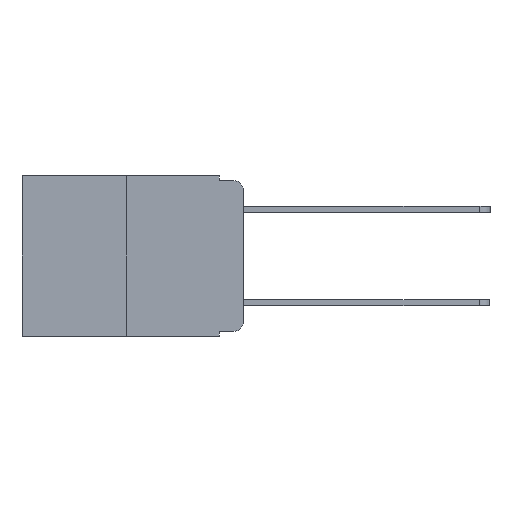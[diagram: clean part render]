
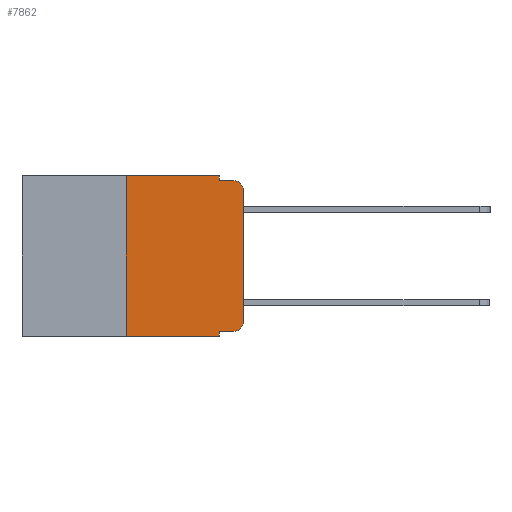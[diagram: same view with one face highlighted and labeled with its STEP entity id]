
A CAD part, left-side view. The second image highlights one B-rep face of the part: STEP entity #7862.
In plain terms, the highlighted planar face has unit normal (-1, 0, 0).
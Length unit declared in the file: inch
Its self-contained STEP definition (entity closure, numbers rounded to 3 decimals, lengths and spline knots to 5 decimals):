
#88 = ORIENTED_EDGE ( 'NONE', *, *, #5108, .T. ) ;
#132 = CARTESIAN_POINT ( 'NONE',  ( 0., 0.02, -0.01 ) ) ;
#271 = VERTEX_POINT ( 'NONE', #17676 ) ;
#285 = LINE ( 'NONE', #19377, #10182 ) ;
#403 = CARTESIAN_POINT ( 'NONE',  ( 0., 0.25, 0. ) ) ;
#944 = VECTOR ( 'NONE', #24253, 39.37008 ) ;
#967 = LINE ( 'NONE', #19892, #7755 ) ;
#1356 = CARTESIAN_POINT ( 'NONE',  ( 0., 0.051, 0. ) ) ;
#1416 = CIRCLE ( 'NONE', #23635, 0.02 ) ;
#1637 = CARTESIAN_POINT ( 'NONE',  ( 0., 0.02, -0.03 ) ) ;
#1707 = DIRECTION ( 'NONE',  ( 0., -1., 0. ) ) ;
#1805 = VERTEX_POINT ( 'NONE', #12002 ) ;
#2057 = CARTESIAN_POINT ( 'NONE',  ( 0., 0.25, -0.343 ) ) ;
#2351 = DIRECTION ( 'NONE',  ( 0., -1., 0. ) ) ;
#2490 = VERTEX_POINT ( 'NONE', #21714 ) ;
#2583 = CARTESIAN_POINT ( 'NONE',  ( 0., 0.473, 0. ) ) ;
#2915 = VERTEX_POINT ( 'NONE', #132 ) ;
#2989 = EDGE_CURVE ( 'NONE', #1805, #16256, #3990, .T. ) ;
#3214 = VERTEX_POINT ( 'NONE', #21107 ) ;
#3270 = ORIENTED_EDGE ( 'NONE', *, *, #4165, .F. ) ;
#3385 = VECTOR ( 'NONE', #1707, 39.37008 ) ;
#3662 = DIRECTION ( 'NONE',  ( 0., 0., -1. ) ) ;
#3990 = LINE ( 'NONE', #11478, #3385 ) ;
#4165 = EDGE_CURVE ( 'NONE', #3214, #9119, #20747, .T. ) ;
#4185 = AXIS2_PLACEMENT_3D ( 'NONE', #1637, #15218, #3662 ) ;
#4324 = EDGE_CURVE ( 'NONE', #1805, #4409, #967, .T. ) ;
#4409 = VERTEX_POINT ( 'NONE', #9359 ) ;
#5108 = EDGE_CURVE ( 'NONE', #10859, #2490, #285, .T. ) ;
#6042 = EDGE_LOOP ( 'NONE', ( #88, #7217, #12386, #22793, #3270, #14163, #10894, #15927, #12108, #21958 ) ) ;
#6493 = FACE_OUTER_BOUND ( 'NONE', #6042, .T. ) ;
#6657 = VECTOR ( 'NONE', #21418, 39.37008 ) ;
#6809 = DIRECTION ( 'NONE',  ( 0., 0., 1. ) ) ;
#6820 = VECTOR ( 'NONE', #2351, 39.37008 ) ;
#7139 = DIRECTION ( 'NONE',  ( 0., 0., -1. ) ) ;
#7217 = ORIENTED_EDGE ( 'NONE', *, *, #22081, .T. ) ;
#7258 = CARTESIAN_POINT ( 'NONE',  ( 0., 0.02, -0.313 ) ) ;
#7755 = VECTOR ( 'NONE', #22128, 39.37008 ) ;
#7862 = ADVANCED_FACE ( 'NONE', ( #6493 ), #19528, .F. ) ;
#9119 = VERTEX_POINT ( 'NONE', #1356 ) ;
#9254 = DIRECTION ( 'NONE',  ( 0., 0., -1. ) ) ;
#9325 = VERTEX_POINT ( 'NONE', #2057 ) ;
#9359 = CARTESIAN_POINT ( 'NONE',  ( 0., 0.051, -0.343 ) ) ;
#9386 = CARTESIAN_POINT ( 'NONE',  ( 0., 0.051, -0.01 ) ) ;
#10182 = VECTOR ( 'NONE', #6809, 39.37008 ) ;
#10185 = DIRECTION ( 'NONE',  ( 1., 0., 0. ) ) ;
#10850 = EDGE_CURVE ( 'NONE', #9325, #3214, #11871, .T. ) ;
#10859 = VERTEX_POINT ( 'NONE', #21501 ) ;
#10894 = ORIENTED_EDGE ( 'NONE', *, *, #22531, .T. ) ;
#10960 = CARTESIAN_POINT ( 'NONE',  ( 0., 0.473, -0.343 ) ) ;
#11478 = CARTESIAN_POINT ( 'NONE',  ( 0., 0.051, -0.333 ) ) ;
#11871 = LINE ( 'NONE', #403, #6657 ) ;
#12002 = CARTESIAN_POINT ( 'NONE',  ( 0., 0.051, -0.333 ) ) ;
#12108 = ORIENTED_EDGE ( 'NONE', *, *, #2989, .T. ) ;
#12386 = ORIENTED_EDGE ( 'NONE', *, *, #19630, .F. ) ;
#12399 = VECTOR ( 'NONE', #7139, 39.37008 ) ;
#14163 = ORIENTED_EDGE ( 'NONE', *, *, #10850, .F. ) ;
#14689 = DIRECTION ( 'NONE',  ( 0., -1., 0. ) ) ;
#15170 = LINE ( 'NONE', #10960, #19516 ) ;
#15218 = DIRECTION ( 'NONE',  ( -1., 0., 0. ) ) ;
#15806 = CARTESIAN_POINT ( 'NONE',  ( 0., 0.473, 0. ) ) ;
#15927 = ORIENTED_EDGE ( 'NONE', *, *, #4324, .F. ) ;
#16256 = VERTEX_POINT ( 'NONE', #24331 ) ;
#17397 = LINE ( 'NONE', #18540, #12399 ) ;
#17676 = CARTESIAN_POINT ( 'NONE',  ( 0., 0.051, -0.01 ) ) ;
#18426 = EDGE_CURVE ( 'NONE', #9119, #271, #17397, .T. ) ;
#18540 = CARTESIAN_POINT ( 'NONE',  ( 0., 0.051, 0. ) ) ;
#19331 = AXIS2_PLACEMENT_3D ( 'NONE', #15806, #10185, #23153 ) ;
#19377 = CARTESIAN_POINT ( 'NONE',  ( 0., 0., 0. ) ) ;
#19499 = CIRCLE ( 'NONE', #4185, 0.02 ) ;
#19516 = VECTOR ( 'NONE', #14689, 39.37008 ) ;
#19528 = PLANE ( 'NONE',  #19331 ) ;
#19630 = EDGE_CURVE ( 'NONE', #271, #2915, #21291, .T. ) ;
#19892 = CARTESIAN_POINT ( 'NONE',  ( 0., 0.051, 0. ) ) ;
#20503 = DIRECTION ( 'NONE',  ( -1., 0., 0. ) ) ;
#20747 = LINE ( 'NONE', #2583, #6820 ) ;
#21107 = CARTESIAN_POINT ( 'NONE',  ( 0., 0.25, 0. ) ) ;
#21291 = LINE ( 'NONE', #9386, #944 ) ;
#21418 = DIRECTION ( 'NONE',  ( 0., 0., 1. ) ) ;
#21501 = CARTESIAN_POINT ( 'NONE',  ( 0., 0., -0.313 ) ) ;
#21714 = CARTESIAN_POINT ( 'NONE',  ( 0., 0., -0.03 ) ) ;
#21958 = ORIENTED_EDGE ( 'NONE', *, *, #23702, .T. ) ;
#22081 = EDGE_CURVE ( 'NONE', #2490, #2915, #19499, .T. ) ;
#22128 = DIRECTION ( 'NONE',  ( 0., 0., -1. ) ) ;
#22531 = EDGE_CURVE ( 'NONE', #9325, #4409, #15170, .T. ) ;
#22793 = ORIENTED_EDGE ( 'NONE', *, *, #18426, .F. ) ;
#23153 = DIRECTION ( 'NONE',  ( 0., 0., -1. ) ) ;
#23635 = AXIS2_PLACEMENT_3D ( 'NONE', #7258, #20503, #9254 ) ;
#23702 = EDGE_CURVE ( 'NONE', #16256, #10859, #1416, .T. ) ;
#24253 = DIRECTION ( 'NONE',  ( 0., -1., 0. ) ) ;
#24331 = CARTESIAN_POINT ( 'NONE',  ( 0., 0.02, -0.333 ) ) ;
